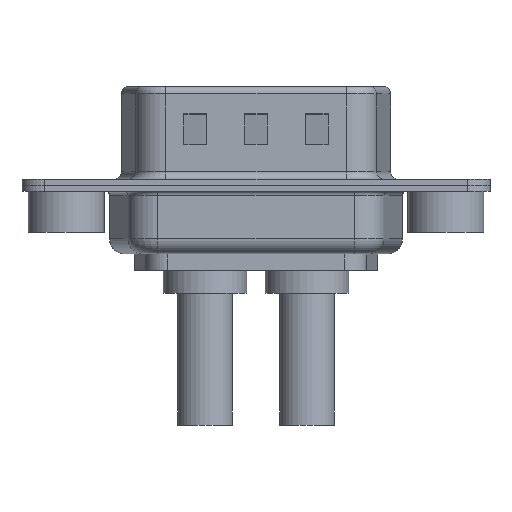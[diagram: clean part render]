
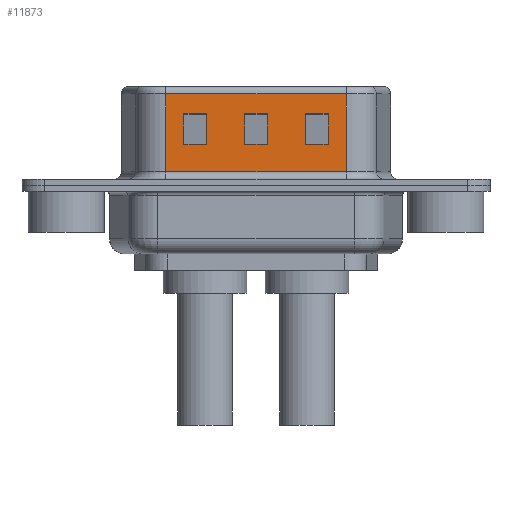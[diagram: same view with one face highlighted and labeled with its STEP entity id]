
A CAD part, front view. The second image highlights one B-rep face of the part: STEP entity #11873.
In plain terms, the highlighted planar face has unit normal (0, -1, 0).
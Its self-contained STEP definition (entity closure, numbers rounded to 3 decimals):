
#21 = EDGE_LOOP ( 'NONE', ( #6629, #9836, #12730, #14926 ) ) ;
#41 = VECTOR ( 'NONE', #4527, 1000. ) ;
#53 = LINE ( 'NONE', #3184, #14043 ) ;
#180 = VERTEX_POINT ( 'NONE', #16659 ) ;
#262 = LINE ( 'NONE', #2680, #6251 ) ;
#351 = CARTESIAN_POINT ( 'NONE',  ( 6.55, -4.58, 6.52 ) ) ;
#536 = LINE ( 'NONE', #4381, #7400 ) ;
#571 = CARTESIAN_POINT ( 'NONE',  ( 15.75, -4.58, 2.705 ) ) ;
#758 = VERTEX_POINT ( 'NONE', #4160 ) ;
#843 = CARTESIAN_POINT ( 'NONE',  ( 9.25, -4.58, 6.52 ) ) ;
#845 = CARTESIAN_POINT ( 'NONE',  ( 6.55, -4.58, 6.02 ) ) ;
#990 = ORIENTED_EDGE ( 'NONE', *, *, #9249, .T. ) ;
#1400 = EDGE_CURVE ( 'NONE', #6558, #180, #7784, .T. ) ;
#1785 = VERTEX_POINT ( 'NONE', #8071 ) ;
#1882 = CARTESIAN_POINT ( 'NONE',  ( 22.45, -4.58, 2.705 ) ) ;
#2042 = ORIENTED_EDGE ( 'NONE', *, *, #7776, .T. ) ;
#2296 = VERTEX_POINT ( 'NONE', #6245 ) ;
#2314 = VECTOR ( 'NONE', #10766, 1000. ) ;
#2604 = EDGE_CURVE ( 'NONE', #180, #3167, #262, .T. ) ;
#2680 = CARTESIAN_POINT ( 'NONE',  ( 7.75, -4.58, 6.52 ) ) ;
#2835 = ORIENTED_EDGE ( 'NONE', *, *, #10547, .T. ) ;
#2867 = EDGE_CURVE ( 'NONE', #12117, #7878, #6871, .T. ) ;
#3029 = FACE_BOUND ( 'NONE', #5891, .T. ) ;
#3149 = ORIENTED_EDGE ( 'NONE', *, *, #16391, .T. ) ;
#3167 = VERTEX_POINT ( 'NONE', #4892 ) ;
#3184 = CARTESIAN_POINT ( 'NONE',  ( 18.45, -4.58, 2.705 ) ) ;
#3204 = EDGE_CURVE ( 'NONE', #3167, #758, #10219, .T. ) ;
#3223 = DIRECTION ( 'NONE',  ( 0., 0., 1. ) ) ;
#3235 = ORIENTED_EDGE ( 'NONE', *, *, #2604, .T. ) ;
#3350 = AXIS2_PLACEMENT_3D ( 'NONE', #16720, #11422, #3223 ) ;
#3531 = VERTEX_POINT ( 'NONE', #12690 ) ;
#3568 = DIRECTION ( 'NONE',  ( 0., 0., 1. ) ) ;
#3571 = CARTESIAN_POINT ( 'NONE',  ( 17.25, -4.58, 4.705 ) ) ;
#3702 = CARTESIAN_POINT ( 'NONE',  ( 18.45, -4.58, 0.9 ) ) ;
#3745 = LINE ( 'NONE', #5116, #7007 ) ;
#3861 = EDGE_CURVE ( 'NONE', #11735, #1785, #536, .T. ) ;
#4160 = CARTESIAN_POINT ( 'NONE',  ( 9.25, -4.58, 4.705 ) ) ;
#4381 = CARTESIAN_POINT ( 'NONE',  ( 18.45, -4.58, 4.705 ) ) ;
#4422 = CARTESIAN_POINT ( 'NONE',  ( 17.25, -4.58, 6.52 ) ) ;
#4527 = DIRECTION ( 'NONE',  ( 0., 0., -1. ) ) ;
#4566 = PLANE ( 'NONE',  #3350 ) ;
#4892 = CARTESIAN_POINT ( 'NONE',  ( 7.75, -4.58, 4.705 ) ) ;
#4926 = VERTEX_POINT ( 'NONE', #13148 ) ;
#5116 = CARTESIAN_POINT ( 'NONE',  ( 18.45, -4.58, 0.9 ) ) ;
#5168 = DIRECTION ( 'NONE',  ( 1., 0., 0. ) ) ;
#5237 = VERTEX_POINT ( 'NONE', #7900 ) ;
#5340 = DIRECTION ( 'NONE',  ( 1., 0., 0. ) ) ;
#5782 = EDGE_CURVE ( 'NONE', #2296, #7067, #16738, .T. ) ;
#5891 = EDGE_LOOP ( 'NONE', ( #2042, #990, #6678, #7840 ) ) ;
#6168 = CARTESIAN_POINT ( 'NONE',  ( 18.45, -4.58, 6.02 ) ) ;
#6245 = CARTESIAN_POINT ( 'NONE',  ( 18.45, -4.58, 6.02 ) ) ;
#6251 = VECTOR ( 'NONE', #13228, 1000. ) ;
#6558 = VERTEX_POINT ( 'NONE', #10078 ) ;
#6629 = ORIENTED_EDGE ( 'NONE', *, *, #3861, .T. ) ;
#6678 = ORIENTED_EDGE ( 'NONE', *, *, #15213, .T. ) ;
#6733 = EDGE_CURVE ( 'NONE', #758, #6558, #10630, .T. ) ;
#6749 = FACE_OUTER_BOUND ( 'NONE', #7789, .T. ) ;
#6787 = DIRECTION ( 'NONE',  ( 1., 0., 0. ) ) ;
#6846 = DIRECTION ( 'NONE',  ( -1., 0., 0. ) ) ;
#6871 = LINE ( 'NONE', #351, #41 ) ;
#7007 = VECTOR ( 'NONE', #5168, 1000. ) ;
#7016 = CARTESIAN_POINT ( 'NONE',  ( 13.25, -4.58, 6.52 ) ) ;
#7067 = VERTEX_POINT ( 'NONE', #3702 ) ;
#7320 = DIRECTION ( 'NONE',  ( 0., 0., -1. ) ) ;
#7400 = VECTOR ( 'NONE', #6787, 1000. ) ;
#7408 = DIRECTION ( 'NONE',  ( -1., 0., 0. ) ) ;
#7435 = CARTESIAN_POINT ( 'NONE',  ( 6.55, -4.58, 0.9 ) ) ;
#7776 = EDGE_CURVE ( 'NONE', #14630, #9766, #12177, .T. ) ;
#7784 = LINE ( 'NONE', #13645, #10880 ) ;
#7789 = EDGE_LOOP ( 'NONE', ( #12861, #3149, #16433, #2835 ) ) ;
#7840 = ORIENTED_EDGE ( 'NONE', *, *, #10789, .T. ) ;
#7878 = VERTEX_POINT ( 'NONE', #7435 ) ;
#7900 = CARTESIAN_POINT ( 'NONE',  ( 11.75, -4.58, 2.705 ) ) ;
#8068 = VECTOR ( 'NONE', #11044, 1000. ) ;
#8071 = CARTESIAN_POINT ( 'NONE',  ( 13.25, -4.58, 4.705 ) ) ;
#8405 = LINE ( 'NONE', #13245, #11568 ) ;
#8597 = VERTEX_POINT ( 'NONE', #571 ) ;
#9249 = EDGE_CURVE ( 'NONE', #9766, #8597, #12750, .T. ) ;
#9328 = VECTOR ( 'NONE', #11065, 1000. ) ;
#9330 = EDGE_CURVE ( 'NONE', #5237, #11735, #14584, .T. ) ;
#9766 = VERTEX_POINT ( 'NONE', #11688 ) ;
#9785 = VECTOR ( 'NONE', #5340, 1000. ) ;
#9801 = VECTOR ( 'NONE', #11767, 1000. ) ;
#9836 = ORIENTED_EDGE ( 'NONE', *, *, #10008, .T. ) ;
#10008 = EDGE_CURVE ( 'NONE', #1785, #4926, #12933, .T. ) ;
#10078 = CARTESIAN_POINT ( 'NONE',  ( 9.25, -4.58, 2.705 ) ) ;
#10219 = LINE ( 'NONE', #15478, #9785 ) ;
#10465 = LINE ( 'NONE', #6168, #13664 ) ;
#10547 = EDGE_CURVE ( 'NONE', #7878, #7067, #3745, .T. ) ;
#10630 = LINE ( 'NONE', #843, #9801 ) ;
#10766 = DIRECTION ( 'NONE',  ( 0., 0., -1. ) ) ;
#10789 = EDGE_CURVE ( 'NONE', #3531, #14630, #11651, .T. ) ;
#10880 = VECTOR ( 'NONE', #6846, 1000. ) ;
#11010 = ORIENTED_EDGE ( 'NONE', *, *, #1400, .T. ) ;
#11033 = VECTOR ( 'NONE', #3568, 1000. ) ;
#11044 = DIRECTION ( 'NONE',  ( 1., 0., 0. ) ) ;
#11065 = DIRECTION ( 'NONE',  ( 0., 0., -1. ) ) ;
#11422 = DIRECTION ( 'NONE',  ( 0., 1., 0. ) ) ;
#11456 = DIRECTION ( 'NONE',  ( -1., 0., 0. ) ) ;
#11568 = VECTOR ( 'NONE', #17150, 1000. ) ;
#11651 = LINE ( 'NONE', #13738, #8068 ) ;
#11688 = CARTESIAN_POINT ( 'NONE',  ( 17.25, -4.58, 2.705 ) ) ;
#11735 = VERTEX_POINT ( 'NONE', #12460 ) ;
#11739 = ORIENTED_EDGE ( 'NONE', *, *, #6733, .T. ) ;
#11767 = DIRECTION ( 'NONE',  ( 0., 0., -1. ) ) ;
#11873 = ADVANCED_FACE ( 'NONE', ( #17386, #3029, #14313, #6749 ), #4566, .F. ) ;
#12117 = VERTEX_POINT ( 'NONE', #845 ) ;
#12177 = LINE ( 'NONE', #4422, #15250 ) ;
#12460 = CARTESIAN_POINT ( 'NONE',  ( 11.75, -4.58, 4.705 ) ) ;
#12690 = CARTESIAN_POINT ( 'NONE',  ( 15.75, -4.58, 4.705 ) ) ;
#12730 = ORIENTED_EDGE ( 'NONE', *, *, #16995, .T. ) ;
#12746 = CARTESIAN_POINT ( 'NONE',  ( 18.45, -4.58, 6.52 ) ) ;
#12750 = LINE ( 'NONE', #1882, #16238 ) ;
#12861 = ORIENTED_EDGE ( 'NONE', *, *, #5782, .F. ) ;
#12933 = LINE ( 'NONE', #7016, #9328 ) ;
#13127 = CARTESIAN_POINT ( 'NONE',  ( 11.75, -4.58, 6.52 ) ) ;
#13148 = CARTESIAN_POINT ( 'NONE',  ( 13.25, -4.58, 2.705 ) ) ;
#13228 = DIRECTION ( 'NONE',  ( 0., 0., 1. ) ) ;
#13245 = CARTESIAN_POINT ( 'NONE',  ( 15.75, -4.58, 6.52 ) ) ;
#13645 = CARTESIAN_POINT ( 'NONE',  ( 14.45, -4.58, 2.705 ) ) ;
#13664 = VECTOR ( 'NONE', #15524, 1000. ) ;
#13738 = CARTESIAN_POINT ( 'NONE',  ( 22.45, -4.58, 4.705 ) ) ;
#14043 = VECTOR ( 'NONE', #7408, 1000. ) ;
#14313 = FACE_BOUND ( 'NONE', #21, .T. ) ;
#14584 = LINE ( 'NONE', #13127, #11033 ) ;
#14630 = VERTEX_POINT ( 'NONE', #3571 ) ;
#14926 = ORIENTED_EDGE ( 'NONE', *, *, #9330, .T. ) ;
#15213 = EDGE_CURVE ( 'NONE', #8597, #3531, #8405, .T. ) ;
#15250 = VECTOR ( 'NONE', #7320, 1000. ) ;
#15478 = CARTESIAN_POINT ( 'NONE',  ( 14.45, -4.58, 4.705 ) ) ;
#15524 = DIRECTION ( 'NONE',  ( -1., 0., 0. ) ) ;
#15704 = EDGE_LOOP ( 'NONE', ( #11739, #11010, #3235, #15872 ) ) ;
#15872 = ORIENTED_EDGE ( 'NONE', *, *, #3204, .T. ) ;
#16238 = VECTOR ( 'NONE', #11456, 1000. ) ;
#16391 = EDGE_CURVE ( 'NONE', #2296, #12117, #10465, .T. ) ;
#16433 = ORIENTED_EDGE ( 'NONE', *, *, #2867, .T. ) ;
#16659 = CARTESIAN_POINT ( 'NONE',  ( 7.75, -4.58, 2.705 ) ) ;
#16720 = CARTESIAN_POINT ( 'NONE',  ( 18.45, -4.58, 6.52 ) ) ;
#16738 = LINE ( 'NONE', #12746, #2314 ) ;
#16995 = EDGE_CURVE ( 'NONE', #4926, #5237, #53, .T. ) ;
#17150 = DIRECTION ( 'NONE',  ( 0., 0., 1. ) ) ;
#17386 = FACE_BOUND ( 'NONE', #15704, .T. ) ;
